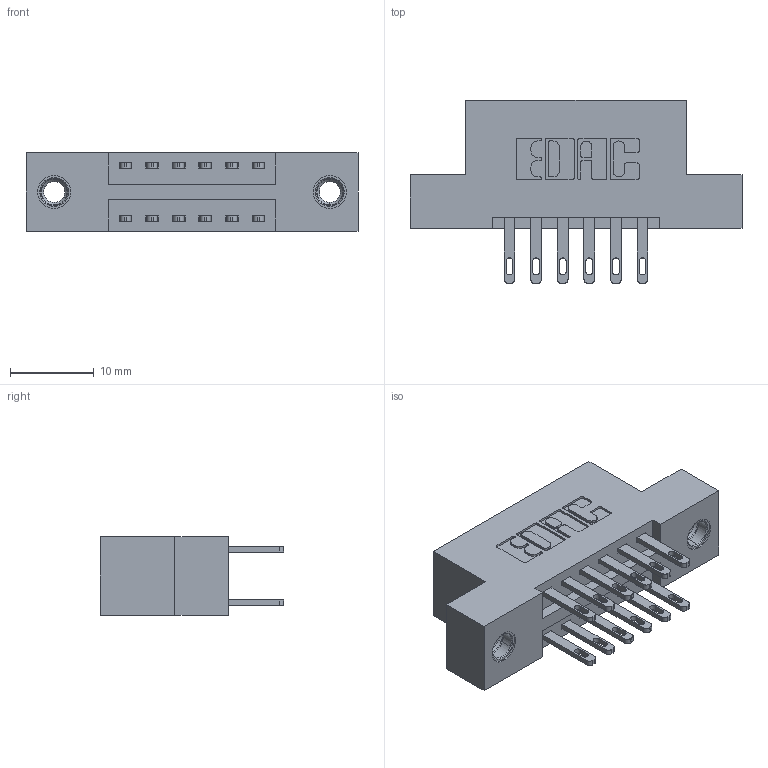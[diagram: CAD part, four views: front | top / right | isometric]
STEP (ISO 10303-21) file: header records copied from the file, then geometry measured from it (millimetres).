
FILE_DESCRIPTION (( 'STEP AP203' ), '1' );
FILE_NAME ('896-012-500-207.STEP', '2021-07-27T14:47:13', ( '' ), ( '' ), 'SwSTEP 2.0', 'SolidWorks 2020', '' );
FILE_SCHEMA (( 'CONFIG_CONTROL_DESIGN' ));
Length unit declared in the file: inch
Products named in the file (4): 846 Part_Flush Mounting Lugs - 0.156 Dia-TI; 345-292-001_345-293-100; 896-012-500-207; 345-250-001_345-250-005-103
Assembly tree (15 placements, depth 2):
  896-012-500-207
    846 Part_Flush Mounting Lugs - 0.156 Dia-TI
    345-292-001_345-293-100  x12
    345-250-001_345-250-005-103  x2
Bounding box: 39.62 x 21.84 x 9.4 mm (x, y, z)
Volume: 3607.4 mm3; surface area: 4552.1 mm2
Topology: 15 solids, 15 shells, 758 faces, 2229 edges, 1478 vertices
Faces by surface type: plane 456, cylinder 286, cone 12, torus 4
Entity records: 9878 total; most frequent: CARTESIAN_POINT 1659, ORIENTED_EDGE 1586, DIRECTION 1543, EDGE_CURVE 793, VECTOR 613, LINE 613, VERTEX_POINT 524, AXIS2_PLACEMENT_3D 465
